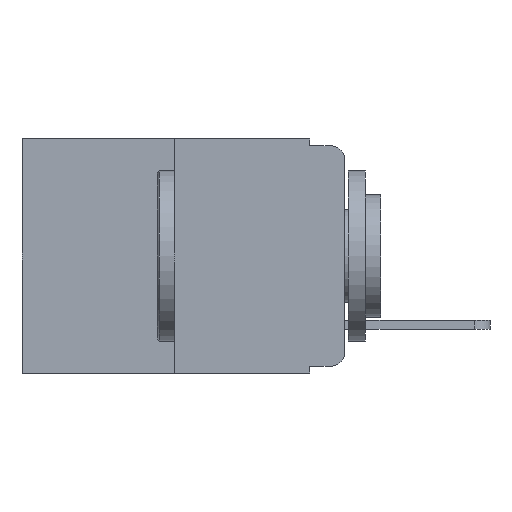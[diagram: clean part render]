
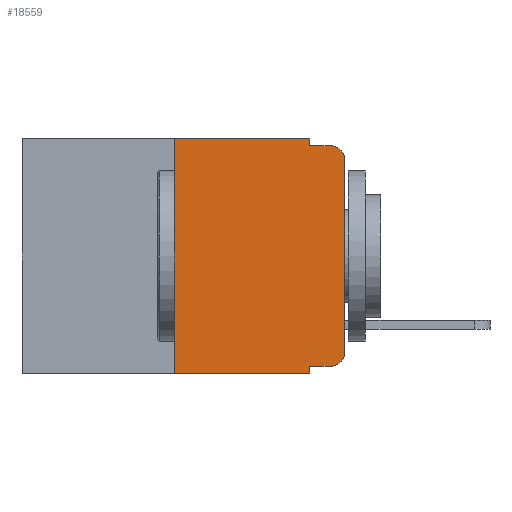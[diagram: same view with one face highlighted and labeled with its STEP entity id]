
A CAD part, left-side view. The second image highlights one B-rep face of the part: STEP entity #18559.
In plain terms, the highlighted planar face has unit normal (-1, 0, 0).
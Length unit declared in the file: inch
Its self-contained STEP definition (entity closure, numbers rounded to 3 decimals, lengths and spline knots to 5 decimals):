
#389 = CIRCLE ( 'NONE', #1973, 0.02 ) ;
#645 = ORIENTED_EDGE ( 'NONE', *, *, #2049, .F. ) ;
#878 = AXIS2_PLACEMENT_3D ( 'NONE', #16646, #3293, #16144 ) ;
#1023 = EDGE_CURVE ( 'NONE', #1187, #14920, #5428, .T. ) ;
#1079 = LINE ( 'NONE', #17107, #17990 ) ;
#1187 = VERTEX_POINT ( 'NONE', #3099 ) ;
#1213 = CARTESIAN_POINT ( 'NONE',  ( 0., 0.051, 0. ) ) ;
#1423 = ORIENTED_EDGE ( 'NONE', *, *, #4884, .F. ) ;
#1727 = EDGE_CURVE ( 'NONE', #15262, #13659, #8750, .T. ) ;
#1973 = AXIS2_PLACEMENT_3D ( 'NONE', #5825, #17253, #18703 ) ;
#2010 = CARTESIAN_POINT ( 'NONE',  ( 0., 0.051, -0.01 ) ) ;
#2049 = EDGE_CURVE ( 'NONE', #15262, #3461, #18002, .T. ) ;
#2335 = VERTEX_POINT ( 'NONE', #1213 ) ;
#2355 = VECTOR ( 'NONE', #16490, 39.37008 ) ;
#2822 = VERTEX_POINT ( 'NONE', #12516 ) ;
#2895 = AXIS2_PLACEMENT_3D ( 'NONE', #8659, #8605, #11505 ) ;
#3099 = CARTESIAN_POINT ( 'NONE',  ( 0., 0.25, -0.343 ) ) ;
#3293 = DIRECTION ( 'NONE',  ( 1., 0., 0. ) ) ;
#3336 = EDGE_LOOP ( 'NONE', ( #16005, #6111, #1423, #13638, #8729, #18324, #5675, #645, #11592, #6288 ) ) ;
#3461 = VERTEX_POINT ( 'NONE', #5678 ) ;
#3920 = EDGE_CURVE ( 'NONE', #13659, #2822, #5755, .T. ) ;
#4552 = DIRECTION ( 'NONE',  ( 0., 0., 1. ) ) ;
#4728 = EDGE_CURVE ( 'NONE', #1187, #3461, #17454, .T. ) ;
#4884 = EDGE_CURVE ( 'NONE', #8680, #18454, #14297, .T. ) ;
#4948 = DIRECTION ( 'NONE',  ( 0., -1., 0. ) ) ;
#5428 = LINE ( 'NONE', #8932, #16248 ) ;
#5675 = ORIENTED_EDGE ( 'NONE', *, *, #4728, .T. ) ;
#5678 = CARTESIAN_POINT ( 'NONE',  ( 0., 0.051, -0.343 ) ) ;
#5755 = CIRCLE ( 'NONE', #2895, 0.02 ) ;
#5825 = CARTESIAN_POINT ( 'NONE',  ( 0., 0.02, -0.03 ) ) ;
#5994 = CARTESIAN_POINT ( 'NONE',  ( 0., 0.02, -0.01 ) ) ;
#6111 = ORIENTED_EDGE ( 'NONE', *, *, #7873, .T. ) ;
#6288 = ORIENTED_EDGE ( 'NONE', *, *, #3920, .T. ) ;
#7059 = DIRECTION ( 'NONE',  ( 0., 0., -1. ) ) ;
#7873 = EDGE_CURVE ( 'NONE', #13187, #18454, #389, .T. ) ;
#7984 = PLANE ( 'NONE',  #878 ) ;
#8605 = DIRECTION ( 'NONE',  ( -1., 0., 0. ) ) ;
#8659 = CARTESIAN_POINT ( 'NONE',  ( 0., 0.02, -0.313 ) ) ;
#8680 = VERTEX_POINT ( 'NONE', #11398 ) ;
#8729 = ORIENTED_EDGE ( 'NONE', *, *, #11471, .F. ) ;
#8750 = LINE ( 'NONE', #13834, #8958 ) ;
#8932 = CARTESIAN_POINT ( 'NONE',  ( 0., 0.25, 0. ) ) ;
#8958 = VECTOR ( 'NONE', #14988, 39.37008 ) ;
#9310 = CARTESIAN_POINT ( 'NONE',  ( 0., 0., -0.03 ) ) ;
#9672 = LINE ( 'NONE', #17299, #15131 ) ;
#10405 = LINE ( 'NONE', #15331, #12001 ) ;
#10424 = CARTESIAN_POINT ( 'NONE',  ( 0., 0.02, -0.333 ) ) ;
#10871 = FACE_OUTER_BOUND ( 'NONE', #3336, .T. ) ;
#11398 = CARTESIAN_POINT ( 'NONE',  ( 0., 0.051, -0.01 ) ) ;
#11471 = EDGE_CURVE ( 'NONE', #14920, #2335, #10405, .T. ) ;
#11505 = DIRECTION ( 'NONE',  ( 0., 0., -1. ) ) ;
#11592 = ORIENTED_EDGE ( 'NONE', *, *, #1727, .T. ) ;
#11906 = DIRECTION ( 'NONE',  ( 0., 0., 1. ) ) ;
#12001 = VECTOR ( 'NONE', #16968, 39.37008 ) ;
#12516 = CARTESIAN_POINT ( 'NONE',  ( 0., 0., -0.313 ) ) ;
#13010 = EDGE_CURVE ( 'NONE', #2822, #13187, #9672, .T. ) ;
#13187 = VERTEX_POINT ( 'NONE', #9310 ) ;
#13260 = VECTOR ( 'NONE', #14596, 39.37008 ) ;
#13638 = ORIENTED_EDGE ( 'NONE', *, *, #14405, .F. ) ;
#13659 = VERTEX_POINT ( 'NONE', #10424 ) ;
#13834 = CARTESIAN_POINT ( 'NONE',  ( 0., 0.051, -0.333 ) ) ;
#14297 = LINE ( 'NONE', #2010, #18122 ) ;
#14405 = EDGE_CURVE ( 'NONE', #2335, #8680, #1079, .T. ) ;
#14596 = DIRECTION ( 'NONE',  ( 0., 0., -1. ) ) ;
#14920 = VERTEX_POINT ( 'NONE', #16077 ) ;
#14988 = DIRECTION ( 'NONE',  ( 0., -1., 0. ) ) ;
#15131 = VECTOR ( 'NONE', #4552, 39.37008 ) ;
#15262 = VERTEX_POINT ( 'NONE', #18013 ) ;
#15331 = CARTESIAN_POINT ( 'NONE',  ( 0., 0.473, 0. ) ) ;
#15970 = CARTESIAN_POINT ( 'NONE',  ( 0., 0.051, 0. ) ) ;
#16005 = ORIENTED_EDGE ( 'NONE', *, *, #13010, .T. ) ;
#16077 = CARTESIAN_POINT ( 'NONE',  ( 0., 0.25, 0. ) ) ;
#16144 = DIRECTION ( 'NONE',  ( 0., 0., -1. ) ) ;
#16248 = VECTOR ( 'NONE', #11906, 39.37008 ) ;
#16490 = DIRECTION ( 'NONE',  ( 0., -1., 0. ) ) ;
#16542 = CARTESIAN_POINT ( 'NONE',  ( 0., 0.473, -0.343 ) ) ;
#16646 = CARTESIAN_POINT ( 'NONE',  ( 0., 0.473, 0. ) ) ;
#16968 = DIRECTION ( 'NONE',  ( 0., -1., 0. ) ) ;
#17107 = CARTESIAN_POINT ( 'NONE',  ( 0., 0.051, 0. ) ) ;
#17253 = DIRECTION ( 'NONE',  ( -1., 0., 0. ) ) ;
#17299 = CARTESIAN_POINT ( 'NONE',  ( 0., 0., 0. ) ) ;
#17454 = LINE ( 'NONE', #16542, #2355 ) ;
#17990 = VECTOR ( 'NONE', #7059, 39.37008 ) ;
#18002 = LINE ( 'NONE', #15970, #13260 ) ;
#18013 = CARTESIAN_POINT ( 'NONE',  ( 0., 0.051, -0.333 ) ) ;
#18122 = VECTOR ( 'NONE', #4948, 39.37008 ) ;
#18324 = ORIENTED_EDGE ( 'NONE', *, *, #1023, .F. ) ;
#18454 = VERTEX_POINT ( 'NONE', #5994 ) ;
#18559 = ADVANCED_FACE ( 'NONE', ( #10871 ), #7984, .F. ) ;
#18703 = DIRECTION ( 'NONE',  ( 0., 0., -1. ) ) ;
